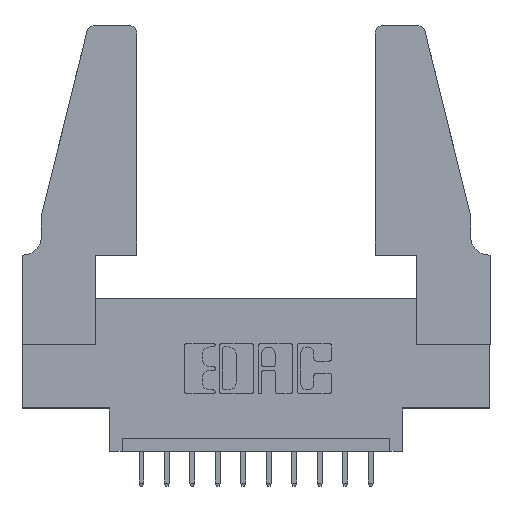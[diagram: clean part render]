
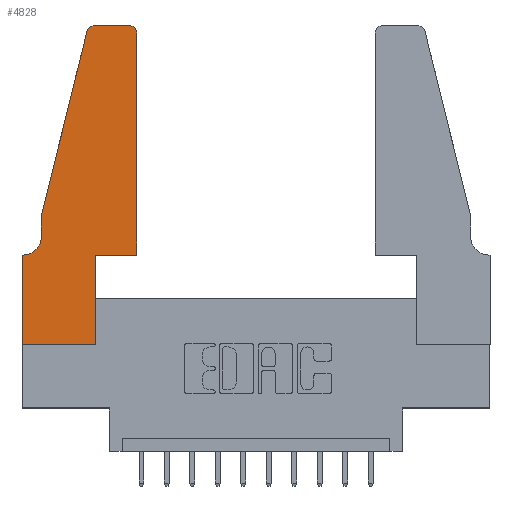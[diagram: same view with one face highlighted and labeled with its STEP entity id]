
A CAD part, top view. The second image highlights one B-rep face of the part: STEP entity #4828.
In plain terms, the highlighted planar face has unit normal (0, 0, 1).
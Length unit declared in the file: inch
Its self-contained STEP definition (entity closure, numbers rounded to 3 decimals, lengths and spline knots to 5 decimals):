
#87 = ORIENTED_EDGE ( 'NONE', *, *, #9279, .T. ) ;
#198 = VERTEX_POINT ( 'NONE', #1376 ) ;
#346 = EDGE_CURVE ( 'NONE', #12081, #720, #8073, .T. ) ;
#377 = LINE ( 'NONE', #444, #3865 ) ;
#420 = EDGE_CURVE ( 'NONE', #1264, #9115, #377, .T. ) ;
#444 = CARTESIAN_POINT ( 'NONE',  ( 0.4505, 0.35, 0.37 ) ) ;
#720 = VERTEX_POINT ( 'NONE', #6628 ) ;
#733 = CARTESIAN_POINT ( 'NONE',  ( 0.4505, 1.22, 0.37 ) ) ;
#949 = EDGE_CURVE ( 'NONE', #9115, #8075, #12112, .T. ) ;
#997 = CARTESIAN_POINT ( 'NONE',  ( 0.0755, 0.42, 0.37 ) ) ;
#1144 = CARTESIAN_POINT ( 'NONE',  ( 0.2865, 0.35, 0.37 ) ) ;
#1264 = VERTEX_POINT ( 'NONE', #7354 ) ;
#1376 = CARTESIAN_POINT ( 'NONE',  ( 0.2865, 0., 0.37 ) ) ;
#1459 = ORIENTED_EDGE ( 'NONE', *, *, #2745, .T. ) ;
#1735 = VERTEX_POINT ( 'NONE', #11786 ) ;
#1764 = EDGE_CURVE ( 'NONE', #198, #1735, #2225, .T. ) ;
#1856 = VECTOR ( 'NONE', #3792, 39.37008 ) ;
#2206 = VERTEX_POINT ( 'NONE', #997 ) ;
#2208 = LINE ( 'NONE', #6600, #7569 ) ;
#2225 = LINE ( 'NONE', #1144, #10290 ) ;
#2237 = EDGE_CURVE ( 'NONE', #720, #198, #2208, .T. ) ;
#2282 = DIRECTION ( 'NONE',  ( 0., 0., 1. ) ) ;
#2477 = DIRECTION ( 'NONE',  ( 0., -1., 0. ) ) ;
#2497 = FACE_OUTER_BOUND ( 'NONE', #4385, .T. ) ;
#2601 = CIRCLE ( 'NONE', #4007, 0.07 ) ;
#2745 = EDGE_CURVE ( 'NONE', #9535, #2206, #12369, .T. ) ;
#2769 = DIRECTION ( 'NONE',  ( 1., 0., 0. ) ) ;
#3066 = DIRECTION ( 'NONE',  ( 0., 0., 1. ) ) ;
#3333 = ORIENTED_EDGE ( 'NONE', *, *, #11608, .T. ) ;
#3577 = LINE ( 'NONE', #4716, #1856 ) ;
#3792 = DIRECTION ( 'NONE',  ( -1., 0., 0. ) ) ;
#3865 = VECTOR ( 'NONE', #8144, 39.37008 ) ;
#3965 = EDGE_CURVE ( 'NONE', #8075, #7763, #3577, .T. ) ;
#4007 = AXIS2_PLACEMENT_3D ( 'NONE', #12242, #13331, #9952 ) ;
#4162 = AXIS2_PLACEMENT_3D ( 'NONE', #10174, #11251, #9258 ) ;
#4340 = DIRECTION ( 'NONE',  ( 0., 1., 0. ) ) ;
#4385 = EDGE_LOOP ( 'NONE', ( #6887, #13090, #3333, #1459, #9838, #11187, #12731, #4552, #6167, #87, #10030, #9028 ) ) ;
#4549 = VECTOR ( 'NONE', #11649, 39.37008 ) ;
#4552 = ORIENTED_EDGE ( 'NONE', *, *, #2237, .T. ) ;
#4716 = CARTESIAN_POINT ( 'NONE',  ( 0.2605, 1.25, 0.37 ) ) ;
#4745 = EDGE_CURVE ( 'NONE', #6455, #12081, #10038, .T. ) ;
#4828 = ADVANCED_FACE ( 'NONE', ( #2497 ), #6881, .T. ) ;
#4919 = DIRECTION ( 'NONE',  ( 1., 0., 0. ) ) ;
#5914 = CARTESIAN_POINT ( 'NONE',  ( 0., 0., 0.37 ) ) ;
#6064 = CARTESIAN_POINT ( 'NONE',  ( 0.284, 1.22, 0.37 ) ) ;
#6167 = ORIENTED_EDGE ( 'NONE', *, *, #1764, .T. ) ;
#6407 = DIRECTION ( 'NONE',  ( -1., 0., 0. ) ) ;
#6455 = VERTEX_POINT ( 'NONE', #12627 ) ;
#6460 = DIRECTION ( 'NONE',  ( 1., 0., 0. ) ) ;
#6600 = CARTESIAN_POINT ( 'NONE',  ( 0., 0., 0.37 ) ) ;
#6628 = CARTESIAN_POINT ( 'NONE',  ( 0., 0., 0.37 ) ) ;
#6881 = PLANE ( 'NONE',  #4162 ) ;
#6887 = ORIENTED_EDGE ( 'NONE', *, *, #3965, .T. ) ;
#7008 = LINE ( 'NONE', #11372, #10882 ) ;
#7354 = CARTESIAN_POINT ( 'NONE',  ( 0.4505, 0.35, 0.37 ) ) ;
#7380 = EDGE_CURVE ( 'NONE', #7763, #8122, #9698, .T. ) ;
#7569 = VECTOR ( 'NONE', #6460, 39.37008 ) ;
#7754 = CARTESIAN_POINT ( 'NONE',  ( 0.4205, 1.22, 0.37 ) ) ;
#7763 = VERTEX_POINT ( 'NONE', #13583 ) ;
#8073 = LINE ( 'NONE', #5914, #4549 ) ;
#8075 = VERTEX_POINT ( 'NONE', #10312 ) ;
#8122 = VERTEX_POINT ( 'NONE', #13368 ) ;
#8144 = DIRECTION ( 'NONE',  ( 0., 1., 0. ) ) ;
#8162 = VECTOR ( 'NONE', #14005, 39.37008 ) ;
#8374 = EDGE_CURVE ( 'NONE', #2206, #6455, #2601, .T. ) ;
#8787 = AXIS2_PLACEMENT_3D ( 'NONE', #6064, #3066, #2769 ) ;
#9028 = ORIENTED_EDGE ( 'NONE', *, *, #949, .T. ) ;
#9115 = VERTEX_POINT ( 'NONE', #733 ) ;
#9137 = AXIS2_PLACEMENT_3D ( 'NONE', #7754, #2282, #13348 ) ;
#9258 = DIRECTION ( 'NONE',  ( 1., 0., 0. ) ) ;
#9279 = EDGE_CURVE ( 'NONE', #1735, #1264, #7008, .T. ) ;
#9535 = VERTEX_POINT ( 'NONE', #9730 ) ;
#9667 = CARTESIAN_POINT ( 'NONE',  ( 0., 0.35, 0.37 ) ) ;
#9698 = CIRCLE ( 'NONE', #8787, 0.03 ) ;
#9730 = CARTESIAN_POINT ( 'NONE',  ( 0.0755, 0.5, 0.37 ) ) ;
#9838 = ORIENTED_EDGE ( 'NONE', *, *, #8374, .T. ) ;
#9952 = DIRECTION ( 'NONE',  ( -1., 0., 0. ) ) ;
#10030 = ORIENTED_EDGE ( 'NONE', *, *, #420, .T. ) ;
#10038 = LINE ( 'NONE', #14164, #10090 ) ;
#10090 = VECTOR ( 'NONE', #6407, 39.37008 ) ;
#10174 = CARTESIAN_POINT ( 'NONE',  ( 0., 0.35, 0.37 ) ) ;
#10290 = VECTOR ( 'NONE', #4340, 39.37008 ) ;
#10312 = CARTESIAN_POINT ( 'NONE',  ( 0.4205, 1.25, 0.37 ) ) ;
#10882 = VECTOR ( 'NONE', #4919, 39.37008 ) ;
#11187 = ORIENTED_EDGE ( 'NONE', *, *, #4745, .T. ) ;
#11251 = DIRECTION ( 'NONE',  ( 0., 0., 1. ) ) ;
#11372 = CARTESIAN_POINT ( 'NONE',  ( 0.4505, 0.35, 0.37 ) ) ;
#11608 = EDGE_CURVE ( 'NONE', #8122, #9535, #13932, .T. ) ;
#11649 = DIRECTION ( 'NONE',  ( 0., -1., 0. ) ) ;
#11786 = CARTESIAN_POINT ( 'NONE',  ( 0.2865, 0.35, 0.37 ) ) ;
#12081 = VERTEX_POINT ( 'NONE', #9667 ) ;
#12112 = CIRCLE ( 'NONE', #9137, 0.03 ) ;
#12242 = CARTESIAN_POINT ( 'NONE',  ( 0.0055, 0.42, 0.37 ) ) ;
#12369 = LINE ( 'NONE', #12447, #13763 ) ;
#12447 = CARTESIAN_POINT ( 'NONE',  ( 0.0755, 0.5, 0.37 ) ) ;
#12627 = CARTESIAN_POINT ( 'NONE',  ( 0.0055, 0.35, 0.37 ) ) ;
#12731 = ORIENTED_EDGE ( 'NONE', *, *, #346, .T. ) ;
#13090 = ORIENTED_EDGE ( 'NONE', *, *, #7380, .T. ) ;
#13331 = DIRECTION ( 'NONE',  ( 0., 0., -1. ) ) ;
#13348 = DIRECTION ( 'NONE',  ( 1., 0., 0. ) ) ;
#13368 = CARTESIAN_POINT ( 'NONE',  ( 0.25487, 1.22718, 0.37 ) ) ;
#13583 = CARTESIAN_POINT ( 'NONE',  ( 0.284, 1.25, 0.37 ) ) ;
#13763 = VECTOR ( 'NONE', #2477, 39.37008 ) ;
#13792 = CARTESIAN_POINT ( 'NONE',  ( 0.0755, 0.5, 0.37 ) ) ;
#13932 = LINE ( 'NONE', #13792, #8162 ) ;
#14005 = DIRECTION ( 'NONE',  ( -0.239, -0.971, 0. ) ) ;
#14164 = CARTESIAN_POINT ( 'NONE',  ( 0.0755, 0.35, 0.37 ) ) ;
